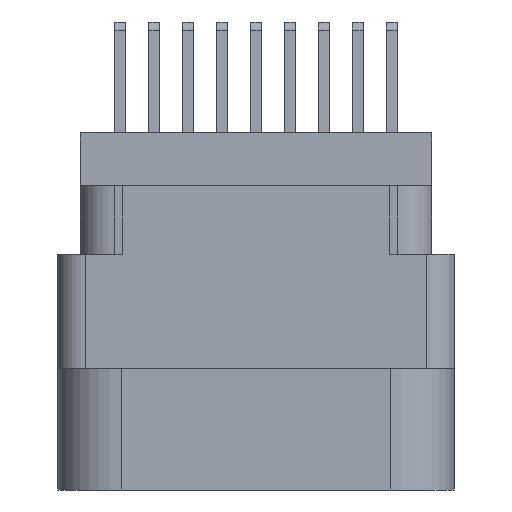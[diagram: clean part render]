
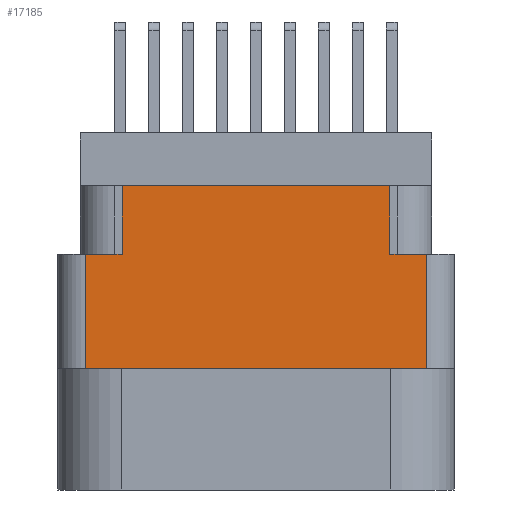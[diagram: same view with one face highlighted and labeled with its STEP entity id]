
A CAD part, left-side view. The second image highlights one B-rep face of the part: STEP entity #17185.
In plain terms, the highlighted planar face has unit normal (-1, 0, 0).
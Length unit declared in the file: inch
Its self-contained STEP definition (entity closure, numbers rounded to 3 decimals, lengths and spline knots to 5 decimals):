
#2144 = AXIS2_PLACEMENT_3D ( 'NONE', #27185, #16432, #4205 ) ;
#2277 = ORIENTED_EDGE ( 'NONE', *, *, #28349, .F. ) ;
#3047 = VECTOR ( 'NONE', #9034, 39.37008 ) ;
#3067 = ORIENTED_EDGE ( 'NONE', *, *, #17535, .T. ) ;
#3967 = CARTESIAN_POINT ( 'NONE',  ( -1., -0.296, -0.268 ) ) ;
#3988 = CARTESIAN_POINT ( 'NONE',  ( -1., 0.296, -0.268 ) ) ;
#4205 = DIRECTION ( 'NONE',  ( 0., 0., 1. ) ) ;
#4628 = VERTEX_POINT ( 'NONE', #9351 ) ;
#4673 = EDGE_CURVE ( 'NONE', #4628, #18111, #28580, .T. ) ;
#6047 = VERTEX_POINT ( 'NONE', #27684 ) ;
#6388 = VERTEX_POINT ( 'NONE', #26808 ) ;
#7420 = CARTESIAN_POINT ( 'NONE',  ( -1., 0.376, -0.52 ) ) ;
#8240 = VERTEX_POINT ( 'NONE', #3967 ) ;
#8241 = CARTESIAN_POINT ( 'NONE',  ( -1., -0.296, -0.268 ) ) ;
#8610 = PLANE ( 'NONE',  #2144 ) ;
#8945 = ORIENTED_EDGE ( 'NONE', *, *, #25657, .T. ) ;
#9034 = DIRECTION ( 'NONE',  ( 0., -1., 0. ) ) ;
#9351 = CARTESIAN_POINT ( 'NONE',  ( -1., -0.376, -0.52 ) ) ;
#10194 = EDGE_CURVE ( 'NONE', #6047, #14709, #27468, .T. ) ;
#10351 = DIRECTION ( 'NONE',  ( 0., 0., 1. ) ) ;
#10857 = EDGE_CURVE ( 'NONE', #14709, #6388, #27765, .T. ) ;
#11863 = EDGE_CURVE ( 'NONE', #6388, #29694, #31749, .T. ) ;
#12328 = ORIENTED_EDGE ( 'NONE', *, *, #10857, .F. ) ;
#14014 = CARTESIAN_POINT ( 'NONE',  ( -1., 0.376, -0.789 ) ) ;
#14709 = VERTEX_POINT ( 'NONE', #3988 ) ;
#15356 = CARTESIAN_POINT ( 'NONE',  ( -1., -0.376, -0.268 ) ) ;
#15449 = CARTESIAN_POINT ( 'NONE',  ( -1., -0.376, -0.789 ) ) ;
#15506 = VECTOR ( 'NONE', #33216, 39.37008 ) ;
#16432 = DIRECTION ( 'NONE',  ( -1., 0., 0. ) ) ;
#16745 = VECTOR ( 'NONE', #21665, 39.37008 ) ;
#16776 = VECTOR ( 'NONE', #17959, 39.37008 ) ;
#17064 = CARTESIAN_POINT ( 'NONE',  ( -1., 0., -0.268 ) ) ;
#17109 = CARTESIAN_POINT ( 'NONE',  ( -1., 0., -0.268 ) ) ;
#17185 = ADVANCED_FACE ( 'NONE', ( #21899 ), #8610, .T. ) ;
#17535 = EDGE_CURVE ( 'NONE', #30499, #4628, #27750, .T. ) ;
#17706 = CARTESIAN_POINT ( 'NONE',  ( -1., -0.296, -0.117 ) ) ;
#17959 = DIRECTION ( 'NONE',  ( 0., -1., 0. ) ) ;
#18111 = VERTEX_POINT ( 'NONE', #15356 ) ;
#18624 = DIRECTION ( 'NONE',  ( 0., 0., 1. ) ) ;
#21665 = DIRECTION ( 'NONE',  ( 0., -1., 0. ) ) ;
#21841 = CARTESIAN_POINT ( 'NONE',  ( -1., 0., -0.52 ) ) ;
#21899 = FACE_OUTER_BOUND ( 'NONE', #27928, .T. ) ;
#22013 = DIRECTION ( 'NONE',  ( 0., 0., -1. ) ) ;
#22136 = VECTOR ( 'NONE', #10351, 39.37008 ) ;
#22726 = ORIENTED_EDGE ( 'NONE', *, *, #11863, .F. ) ;
#22816 = CARTESIAN_POINT ( 'NONE',  ( -1., 0.296, -0.268 ) ) ;
#23513 = VECTOR ( 'NONE', #18624, 39.37008 ) ;
#25657 = EDGE_CURVE ( 'NONE', #6047, #30499, #32253, .T. ) ;
#26106 = ORIENTED_EDGE ( 'NONE', *, *, #32464, .T. ) ;
#26808 = CARTESIAN_POINT ( 'NONE',  ( -1., 0.296, -0.117 ) ) ;
#27185 = CARTESIAN_POINT ( 'NONE',  ( -1., -0.438, -0.789 ) ) ;
#27216 = VECTOR ( 'NONE', #22013, 39.37008 ) ;
#27468 = LINE ( 'NONE', #17064, #31805 ) ;
#27684 = CARTESIAN_POINT ( 'NONE',  ( -1., 0.376, -0.268 ) ) ;
#27750 = LINE ( 'NONE', #21841, #16745 ) ;
#27765 = LINE ( 'NONE', #22816, #15506 ) ;
#27928 = EDGE_LOOP ( 'NONE', ( #29506, #8945, #3067, #32098, #2277, #26106, #22726, #12328 ) ) ;
#28349 = EDGE_CURVE ( 'NONE', #8240, #18111, #30092, .T. ) ;
#28580 = LINE ( 'NONE', #15449, #22136 ) ;
#29506 = ORIENTED_EDGE ( 'NONE', *, *, #10194, .F. ) ;
#29694 = VERTEX_POINT ( 'NONE', #17706 ) ;
#29832 = CARTESIAN_POINT ( 'NONE',  ( -1., 0.438, -0.117 ) ) ;
#30092 = LINE ( 'NONE', #17109, #16776 ) ;
#30499 = VERTEX_POINT ( 'NONE', #7420 ) ;
#31576 = LINE ( 'NONE', #8241, #23513 ) ;
#31749 = LINE ( 'NONE', #29832, #3047 ) ;
#31805 = VECTOR ( 'NONE', #32255, 39.37008 ) ;
#32098 = ORIENTED_EDGE ( 'NONE', *, *, #4673, .T. ) ;
#32253 = LINE ( 'NONE', #14014, #27216 ) ;
#32255 = DIRECTION ( 'NONE',  ( 0., -1., 0. ) ) ;
#32464 = EDGE_CURVE ( 'NONE', #8240, #29694, #31576, .T. ) ;
#33216 = DIRECTION ( 'NONE',  ( 0., 0., 1. ) ) ;
